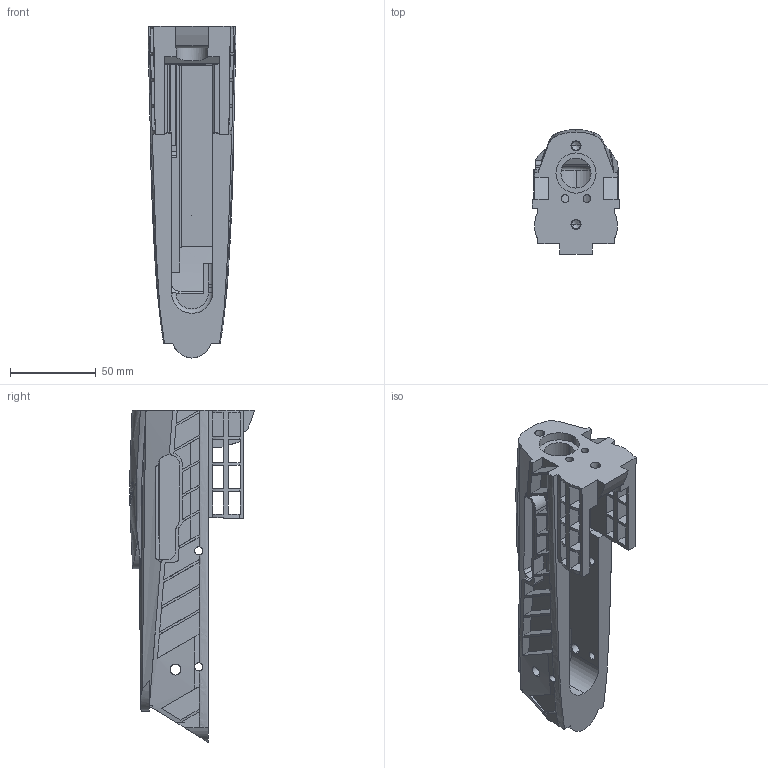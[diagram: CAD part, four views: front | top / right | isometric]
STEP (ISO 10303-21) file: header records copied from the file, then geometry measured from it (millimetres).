
FILE_DESCRIPTION (( 'STEP AP214' ), '1' );
FILE_NAME ('Romulan Charger Receiver v0.5.STEP', '2020-10-11T01:55:13', ( '' ), ( '' ), 'SwSTEP 2.0', 'SolidWorks 2020', '' );
FILE_SCHEMA (( 'AUTOMOTIVE_DESIGN' ));
Length unit declared in the file: inch
Products named in the file (1): Romulan Charger Receiver v0.5
Bounding box: 51.07 x 72.58 x 193.04 mm (x, y, z)
Volume: 181974.1 mm3; surface area: 65370.1 mm2
Topology: 1 solids, 3 shells, 631 faces, 1849 edges, 1202 vertices
Faces by surface type: plane 321, bspline 225, cylinder 68, cone 16, torus 1
Entity records: 32842 total; most frequent: CARTESIAN_POINT 18569, ORIENTED_EDGE 3678, EDGE_CURVE 1839, DIRECTION 1797, VERTEX_POINT 1202, B_SPLINE_CURVE_WITH_KNOTS 925, LINE 763, VECTOR 763
